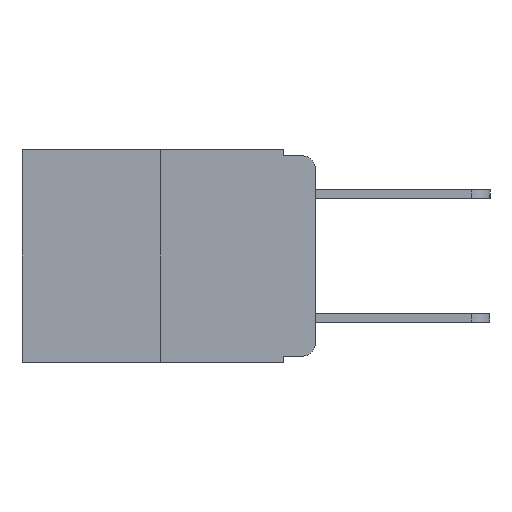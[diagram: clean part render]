
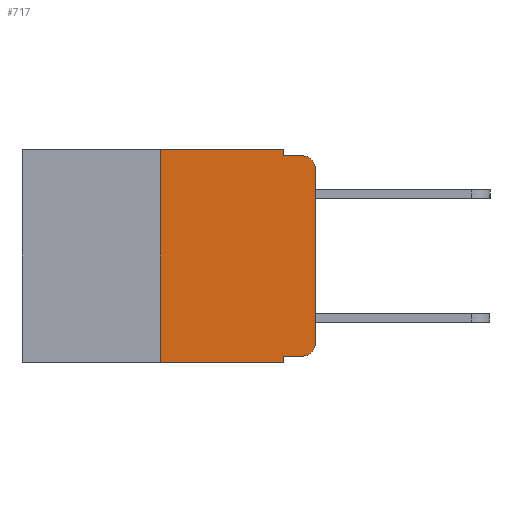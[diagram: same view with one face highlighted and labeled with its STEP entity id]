
A CAD part, left-side view. The second image highlights one B-rep face of the part: STEP entity #717.
In plain terms, the highlighted planar face has unit normal (-1, 0, 0).
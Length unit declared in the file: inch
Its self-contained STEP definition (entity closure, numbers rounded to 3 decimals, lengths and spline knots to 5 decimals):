
#9 = CARTESIAN_POINT ( 'NONE',  ( 0., 0.051, -0.01 ) ) ;
#126 = VECTOR ( 'NONE', #10029, 39.37008 ) ;
#241 = EDGE_CURVE ( 'NONE', #11522, #2878, #7047, .T. ) ;
#291 = VECTOR ( 'NONE', #10314, 39.37008 ) ;
#510 = EDGE_CURVE ( 'NONE', #2878, #3262, #8835, .T. ) ;
#717 = ADVANCED_FACE ( 'NONE', ( #12871 ), #8440, .F. ) ;
#763 = VECTOR ( 'NONE', #4120, 39.37008 ) ;
#833 = VERTEX_POINT ( 'NONE', #1785 ) ;
#1018 = CARTESIAN_POINT ( 'NONE',  ( 0., 0.473, -0.343 ) ) ;
#1508 = EDGE_CURVE ( 'NONE', #5442, #3262, #12519, .T. ) ;
#1605 = VERTEX_POINT ( 'NONE', #3720 ) ;
#1642 = EDGE_CURVE ( 'NONE', #833, #8065, #13276, .T. ) ;
#1693 = EDGE_CURVE ( 'NONE', #6269, #1605, #10131, .T. ) ;
#1785 = CARTESIAN_POINT ( 'NONE',  ( 0., 0.02, -0.333 ) ) ;
#2364 = EDGE_CURVE ( 'NONE', #1605, #11522, #3276, .T. ) ;
#2878 = VERTEX_POINT ( 'NONE', #13385 ) ;
#2933 = CARTESIAN_POINT ( 'NONE',  ( 0., 0.051, -0.333 ) ) ;
#3072 = CARTESIAN_POINT ( 'NONE',  ( 0., 0.25, 0. ) ) ;
#3167 = EDGE_CURVE ( 'NONE', #11519, #833, #8745, .T. ) ;
#3262 = VERTEX_POINT ( 'NONE', #4894 ) ;
#3276 = LINE ( 'NONE', #4990, #11587 ) ;
#3678 = CARTESIAN_POINT ( 'NONE',  ( 0., 0., 0. ) ) ;
#3702 = CARTESIAN_POINT ( 'NONE',  ( 0., 0., -0.03 ) ) ;
#3720 = CARTESIAN_POINT ( 'NONE',  ( 0., 0.25, 0. ) ) ;
#4086 = AXIS2_PLACEMENT_3D ( 'NONE', #5164, #5217, #7272 ) ;
#4102 = ORIENTED_EDGE ( 'NONE', *, *, #12195, .T. ) ;
#4120 = DIRECTION ( 'NONE',  ( 0., 0., -1. ) ) ;
#4501 = ORIENTED_EDGE ( 'NONE', *, *, #1508, .T. ) ;
#4607 = CARTESIAN_POINT ( 'NONE',  ( 0., 0.02, -0.313 ) ) ;
#4648 = VECTOR ( 'NONE', #6469, 39.37008 ) ;
#4839 = ORIENTED_EDGE ( 'NONE', *, *, #510, .F. ) ;
#4875 = DIRECTION ( 'NONE',  ( 0., -1., 0. ) ) ;
#4894 = CARTESIAN_POINT ( 'NONE',  ( 0., 0.02, -0.01 ) ) ;
#4990 = CARTESIAN_POINT ( 'NONE',  ( 0., 0.473, 0. ) ) ;
#5164 = CARTESIAN_POINT ( 'NONE',  ( 0., 0.02, -0.03 ) ) ;
#5217 = DIRECTION ( 'NONE',  ( -1., 0., 0. ) ) ;
#5315 = ORIENTED_EDGE ( 'NONE', *, *, #241, .F. ) ;
#5442 = VERTEX_POINT ( 'NONE', #3702 ) ;
#5579 = ORIENTED_EDGE ( 'NONE', *, *, #2364, .F. ) ;
#5889 = DIRECTION ( 'NONE',  ( 1., 0., 0. ) ) ;
#5929 = VECTOR ( 'NONE', #7561, 39.37008 ) ;
#5984 = ORIENTED_EDGE ( 'NONE', *, *, #1693, .F. ) ;
#6042 = CARTESIAN_POINT ( 'NONE',  ( 0., 0.473, 0. ) ) ;
#6113 = ORIENTED_EDGE ( 'NONE', *, *, #9472, .T. ) ;
#6177 = EDGE_CURVE ( 'NONE', #11519, #6630, #10601, .T. ) ;
#6233 = ORIENTED_EDGE ( 'NONE', *, *, #6177, .F. ) ;
#6269 = VERTEX_POINT ( 'NONE', #9002 ) ;
#6306 = AXIS2_PLACEMENT_3D ( 'NONE', #4607, #9682, #10869 ) ;
#6469 = DIRECTION ( 'NONE',  ( 0., 0., 1. ) ) ;
#6630 = VERTEX_POINT ( 'NONE', #8232 ) ;
#6790 = DIRECTION ( 'NONE',  ( 0., 0., -1. ) ) ;
#7047 = LINE ( 'NONE', #11027, #763 ) ;
#7146 = VECTOR ( 'NONE', #11850, 39.37008 ) ;
#7235 = EDGE_LOOP ( 'NONE', ( #4102, #4501, #4839, #5315, #5579, #5984, #6113, #6233, #7404, #7418 ) ) ;
#7272 = DIRECTION ( 'NONE',  ( 0., 0., -1. ) ) ;
#7404 = ORIENTED_EDGE ( 'NONE', *, *, #3167, .T. ) ;
#7418 = ORIENTED_EDGE ( 'NONE', *, *, #1642, .T. ) ;
#7561 = DIRECTION ( 'NONE',  ( 0., -1., 0. ) ) ;
#8065 = VERTEX_POINT ( 'NONE', #12187 ) ;
#8232 = CARTESIAN_POINT ( 'NONE',  ( 0., 0.051, -0.343 ) ) ;
#8359 = CARTESIAN_POINT ( 'NONE',  ( 0., 0.051, 0. ) ) ;
#8440 = PLANE ( 'NONE',  #13073 ) ;
#8745 = LINE ( 'NONE', #2933, #5929 ) ;
#8835 = LINE ( 'NONE', #9, #291 ) ;
#9002 = CARTESIAN_POINT ( 'NONE',  ( 0., 0.25, -0.343 ) ) ;
#9027 = LINE ( 'NONE', #3678, #126 ) ;
#9449 = CARTESIAN_POINT ( 'NONE',  ( 0., 0.051, 0. ) ) ;
#9472 = EDGE_CURVE ( 'NONE', #6269, #6630, #9817, .T. ) ;
#9682 = DIRECTION ( 'NONE',  ( -1., 0., 0. ) ) ;
#9817 = LINE ( 'NONE', #1018, #7146 ) ;
#10029 = DIRECTION ( 'NONE',  ( 0., 0., 1. ) ) ;
#10131 = LINE ( 'NONE', #3072, #4648 ) ;
#10314 = DIRECTION ( 'NONE',  ( 0., -1., 0. ) ) ;
#10322 = VECTOR ( 'NONE', #12105, 39.37008 ) ;
#10601 = LINE ( 'NONE', #8359, #10322 ) ;
#10869 = DIRECTION ( 'NONE',  ( 0., 0., -1. ) ) ;
#11027 = CARTESIAN_POINT ( 'NONE',  ( 0., 0.051, 0. ) ) ;
#11519 = VERTEX_POINT ( 'NONE', #13253 ) ;
#11522 = VERTEX_POINT ( 'NONE', #9449 ) ;
#11587 = VECTOR ( 'NONE', #4875, 39.37008 ) ;
#11850 = DIRECTION ( 'NONE',  ( 0., -1., 0. ) ) ;
#12105 = DIRECTION ( 'NONE',  ( 0., 0., -1. ) ) ;
#12187 = CARTESIAN_POINT ( 'NONE',  ( 0., 0., -0.313 ) ) ;
#12195 = EDGE_CURVE ( 'NONE', #8065, #5442, #9027, .T. ) ;
#12519 = CIRCLE ( 'NONE', #4086, 0.02 ) ;
#12871 = FACE_OUTER_BOUND ( 'NONE', #7235, .T. ) ;
#13073 = AXIS2_PLACEMENT_3D ( 'NONE', #6042, #5889, #6790 ) ;
#13253 = CARTESIAN_POINT ( 'NONE',  ( 0., 0.051, -0.333 ) ) ;
#13276 = CIRCLE ( 'NONE', #6306, 0.02 ) ;
#13385 = CARTESIAN_POINT ( 'NONE',  ( 0., 0.051, -0.01 ) ) ;
